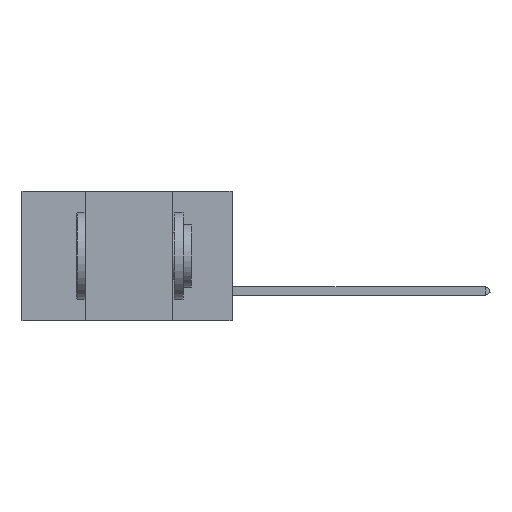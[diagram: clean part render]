
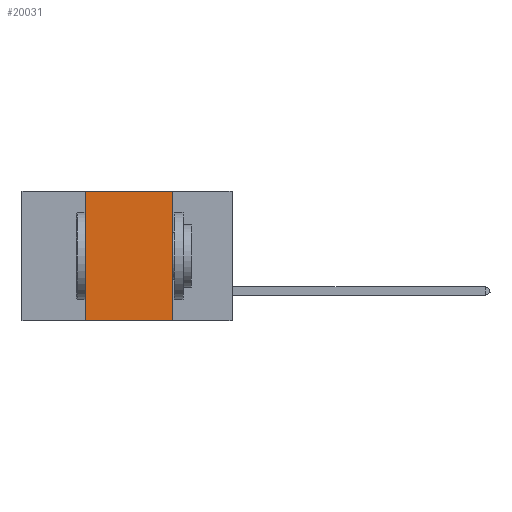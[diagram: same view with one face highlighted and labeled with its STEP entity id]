
A CAD part, left-side view. The second image highlights one B-rep face of the part: STEP entity #20031.
In plain terms, the highlighted planar face has unit normal (-1, 0, 0).
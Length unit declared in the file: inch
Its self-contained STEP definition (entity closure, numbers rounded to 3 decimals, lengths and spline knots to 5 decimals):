
#678 = LINE ( 'NONE', #22736, #22572 ) ;
#2570 = LINE ( 'NONE', #16333, #6729 ) ;
#2832 = PLANE ( 'NONE',  #11617 ) ;
#2987 = CARTESIAN_POINT ( 'NONE',  ( 0., 0.6, -0.37 ) ) ;
#4033 = VERTEX_POINT ( 'NONE', #8527 ) ;
#4102 = VERTEX_POINT ( 'NONE', #5989 ) ;
#4608 = DIRECTION ( 'NONE',  ( 0., -1., 0. ) ) ;
#4689 = ORIENTED_EDGE ( 'NONE', *, *, #21604, .F. ) ;
#5989 = CARTESIAN_POINT ( 'NONE',  ( 0., 0.17, 0. ) ) ;
#6379 = EDGE_CURVE ( 'NONE', #12026, #18938, #18844, .T. ) ;
#6553 = DIRECTION ( 'NONE',  ( 1., 0., 0. ) ) ;
#6729 = VECTOR ( 'NONE', #10948, 39.37008 ) ;
#7987 = ORIENTED_EDGE ( 'NONE', *, *, #22390, .F. ) ;
#8248 = ORIENTED_EDGE ( 'NONE', *, *, #6379, .T. ) ;
#8527 = CARTESIAN_POINT ( 'NONE',  ( 0., 0.42, 0. ) ) ;
#9412 = VECTOR ( 'NONE', #16057, 39.37008 ) ;
#10948 = DIRECTION ( 'NONE',  ( 0., 0., -1. ) ) ;
#11486 = CARTESIAN_POINT ( 'NONE',  ( 0., 0.6, 0. ) ) ;
#11617 = AXIS2_PLACEMENT_3D ( 'NONE', #11486, #6553, #16930 ) ;
#11946 = EDGE_LOOP ( 'NONE', ( #4689, #7987, #13154, #8248 ) ) ;
#12026 = VERTEX_POINT ( 'NONE', #18914 ) ;
#13154 = ORIENTED_EDGE ( 'NONE', *, *, #13416, .F. ) ;
#13416 = EDGE_CURVE ( 'NONE', #12026, #4033, #678, .T. ) ;
#13747 = DIRECTION ( 'NONE',  ( 0., 0., 1. ) ) ;
#14961 = FACE_OUTER_BOUND ( 'NONE', #11946, .T. ) ;
#16057 = DIRECTION ( 'NONE',  ( 0., -1., 0. ) ) ;
#16333 = CARTESIAN_POINT ( 'NONE',  ( 0., 0.17, 0. ) ) ;
#16930 = DIRECTION ( 'NONE',  ( 0., 0., -1. ) ) ;
#18844 = LINE ( 'NONE', #2987, #18874 ) ;
#18874 = VECTOR ( 'NONE', #4608, 39.37008 ) ;
#18914 = CARTESIAN_POINT ( 'NONE',  ( 0., 0.42, -0.37 ) ) ;
#18938 = VERTEX_POINT ( 'NONE', #22169 ) ;
#19621 = LINE ( 'NONE', #21113, #9412 ) ;
#20031 = ADVANCED_FACE ( 'NONE', ( #14961 ), #2832, .F. ) ;
#21113 = CARTESIAN_POINT ( 'NONE',  ( 0., 0.6, 0. ) ) ;
#21604 = EDGE_CURVE ( 'NONE', #4102, #18938, #2570, .T. ) ;
#22169 = CARTESIAN_POINT ( 'NONE',  ( 0., 0.17, -0.37 ) ) ;
#22390 = EDGE_CURVE ( 'NONE', #4033, #4102, #19621, .T. ) ;
#22572 = VECTOR ( 'NONE', #13747, 39.37008 ) ;
#22736 = CARTESIAN_POINT ( 'NONE',  ( 0., 0.42, 0. ) ) ;
